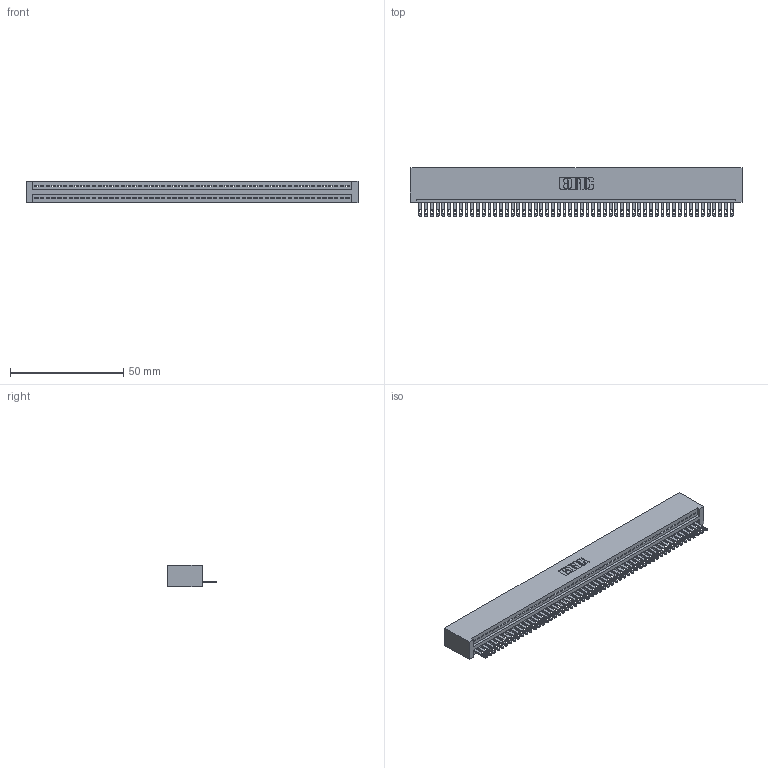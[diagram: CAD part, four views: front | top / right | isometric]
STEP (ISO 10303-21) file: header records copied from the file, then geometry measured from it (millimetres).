
FILE_DESCRIPTION (( 'STEP AP203' ), '1' );
FILE_NAME ('895-055-500-101.STEP', '2020-09-27T14:36:02', ( '' ), ( '' ), 'SwSTEP 2.0', 'SolidWorks 2020', '' );
FILE_SCHEMA (( 'CONFIG_CONTROL_DESIGN' ));
Length unit declared in the file: inch
Products named in the file (3): 845 Part_No Mounting Lugs; 345-292-001_345-293-100; 895-055-500-101
Assembly tree (56 placements, depth 2):
  895-055-500-101
    845 Part_No Mounting Lugs
    345-292-001_345-293-100  x55
Bounding box: 146.3 x 21.51 x 9.4 mm (x, y, z)
Volume: 14621 mm3; surface area: 19920.3 mm2
Topology: 56 solids, 56 shells, 3088 faces, 9557 edges, 6370 vertices
Faces by surface type: plane 1946, cylinder 1142
Entity records: 39297 total; most frequent: CARTESIAN_POINT 6813, ORIENTED_EDGE 6802, DIRECTION 5927, EDGE_CURVE 3401, VECTOR 3053, LINE 3053, VERTEX_POINT 2266, AXIS2_PLACEMENT_3D 1437
